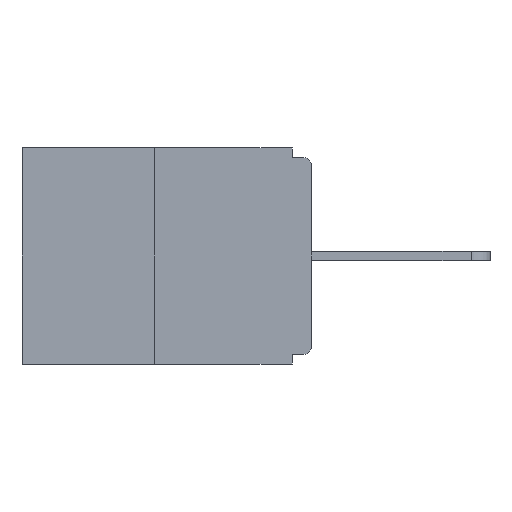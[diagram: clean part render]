
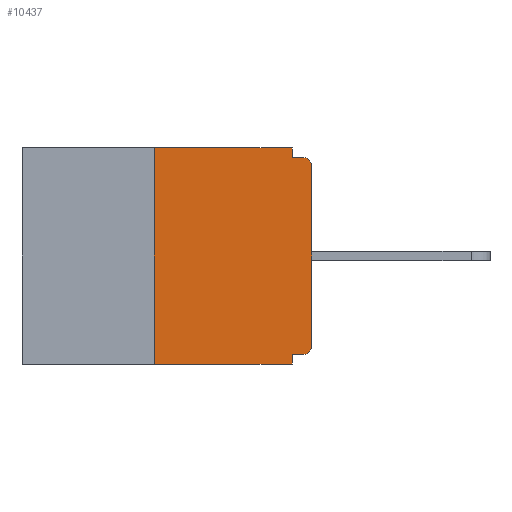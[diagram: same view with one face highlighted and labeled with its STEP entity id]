
A CAD part, left-side view. The second image highlights one B-rep face of the part: STEP entity #10437.
In plain terms, the highlighted planar face has unit normal (-1, 0, 0).
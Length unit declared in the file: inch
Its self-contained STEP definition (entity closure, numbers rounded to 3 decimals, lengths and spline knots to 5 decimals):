
#19 = ORIENTED_EDGE ( 'NONE', *, *, #15145, .T. ) ;
#42 = ORIENTED_EDGE ( 'NONE', *, *, #15051, .T. ) ;
#130 = ORIENTED_EDGE ( 'NONE', *, *, #1402, .F. ) ;
#151 = ORIENTED_EDGE ( 'NONE', *, *, #12578, .F. ) ;
#201 = CARTESIAN_POINT ( 'NONE',  ( 0., 0., -0.03 ) ) ;
#251 = CARTESIAN_POINT ( 'NONE',  ( 0., 0., -0.015 ) ) ;
#617 = VECTOR ( 'NONE', #9192, 39.37008 ) ;
#1059 = ORIENTED_EDGE ( 'NONE', *, *, #19638, .F. ) ;
#1088 = CARTESIAN_POINT ( 'NONE',  ( 0., 0., -0.313 ) ) ;
#1100 = VERTEX_POINT ( 'NONE', #18998 ) ;
#1280 = VERTEX_POINT ( 'NONE', #12153 ) ;
#1402 = EDGE_CURVE ( 'NONE', #17087, #4233, #5703, .T. ) ;
#1859 = DIRECTION ( 'NONE',  ( 0., 0., -1. ) ) ;
#1867 = DIRECTION ( 'NONE',  ( -1., 0., 0. ) ) ;
#1935 = CARTESIAN_POINT ( 'NONE',  ( 0., 0.015, -0.313 ) ) ;
#2205 = CARTESIAN_POINT ( 'NONE',  ( 0., 0.015, -0.03 ) ) ;
#2470 = PLANE ( 'NONE',  #6472 ) ;
#2731 = ORIENTED_EDGE ( 'NONE', *, *, #7790, .T. ) ;
#3092 = CIRCLE ( 'NONE', #11949, 0.015 ) ;
#3506 = CARTESIAN_POINT ( 'NONE',  ( 0., 0.031, 0. ) ) ;
#3685 = VECTOR ( 'NONE', #6808, 39.37008 ) ;
#3762 = EDGE_CURVE ( 'NONE', #1280, #19052, #5853, .T. ) ;
#3929 = DIRECTION ( 'NONE',  ( 0., 0., -1. ) ) ;
#3944 = VECTOR ( 'NONE', #5799, 39.37008 ) ;
#4233 = VERTEX_POINT ( 'NONE', #14925 ) ;
#4263 = DIRECTION ( 'NONE',  ( 0., 0., -1. ) ) ;
#4659 = CARTESIAN_POINT ( 'NONE',  ( 0., 0.25, 0. ) ) ;
#5539 = VERTEX_POINT ( 'NONE', #1088 ) ;
#5685 = LINE ( 'NONE', #17289, #617 ) ;
#5703 = LINE ( 'NONE', #251, #9600 ) ;
#5799 = DIRECTION ( 'NONE',  ( 0., -1., 0. ) ) ;
#5853 = LINE ( 'NONE', #10590, #9749 ) ;
#6281 = VECTOR ( 'NONE', #19668, 39.37008 ) ;
#6472 = AXIS2_PLACEMENT_3D ( 'NONE', #20515, #14186, #4263 ) ;
#6808 = DIRECTION ( 'NONE',  ( 0., 0., -1. ) ) ;
#7246 = CIRCLE ( 'NONE', #17471, 0.015 ) ;
#7374 = EDGE_CURVE ( 'NONE', #8950, #9987, #12668, .T. ) ;
#7462 = CARTESIAN_POINT ( 'NONE',  ( 0., 0.46, 0. ) ) ;
#7615 = LINE ( 'NONE', #3506, #3685 ) ;
#7790 = EDGE_CURVE ( 'NONE', #8950, #20826, #12431, .T. ) ;
#8315 = EDGE_CURVE ( 'NONE', #1280, #5539, #3092, .T. ) ;
#8382 = ORIENTED_EDGE ( 'NONE', *, *, #7374, .F. ) ;
#8950 = VERTEX_POINT ( 'NONE', #19657 ) ;
#9192 = DIRECTION ( 'NONE',  ( 0., 0., 1. ) ) ;
#9600 = VECTOR ( 'NONE', #20470, 39.37008 ) ;
#9749 = VECTOR ( 'NONE', #10820, 39.37008 ) ;
#9987 = VERTEX_POINT ( 'NONE', #4659 ) ;
#10011 = CARTESIAN_POINT ( 'NONE',  ( 0., 0.031, -0.343 ) ) ;
#10437 = ADVANCED_FACE ( 'NONE', ( #19872 ), #2470, .F. ) ;
#10590 = CARTESIAN_POINT ( 'NONE',  ( 0., 0., -0.328 ) ) ;
#10701 = LINE ( 'NONE', #10011, #6281 ) ;
#10724 = ORIENTED_EDGE ( 'NONE', *, *, #21167, .F. ) ;
#10820 = DIRECTION ( 'NONE',  ( 0., 1., 0. ) ) ;
#11164 = VECTOR ( 'NONE', #19238, 39.37008 ) ;
#11949 = AXIS2_PLACEMENT_3D ( 'NONE', #1935, #1867, #1859 ) ;
#11988 = ORIENTED_EDGE ( 'NONE', *, *, #8315, .T. ) ;
#12153 = CARTESIAN_POINT ( 'NONE',  ( 0., 0.015, -0.328 ) ) ;
#12229 = CARTESIAN_POINT ( 'NONE',  ( 0., 0.031, -0.015 ) ) ;
#12431 = LINE ( 'NONE', #18201, #20487 ) ;
#12578 = EDGE_CURVE ( 'NONE', #1100, #17087, #7615, .T. ) ;
#12668 = LINE ( 'NONE', #19597, #11164 ) ;
#13865 = DIRECTION ( 'NONE',  ( -1., 0., 0. ) ) ;
#14186 = DIRECTION ( 'NONE',  ( 1., 0., 0. ) ) ;
#14925 = CARTESIAN_POINT ( 'NONE',  ( 0., 0.015, -0.015 ) ) ;
#15051 = EDGE_CURVE ( 'NONE', #20065, #4233, #7246, .T. ) ;
#15145 = EDGE_CURVE ( 'NONE', #5539, #20065, #5685, .T. ) ;
#15616 = CARTESIAN_POINT ( 'NONE',  ( 0., 0.031, -0.343 ) ) ;
#17070 = LINE ( 'NONE', #7462, #3944 ) ;
#17087 = VERTEX_POINT ( 'NONE', #12229 ) ;
#17289 = CARTESIAN_POINT ( 'NONE',  ( 0., 0., 0. ) ) ;
#17471 = AXIS2_PLACEMENT_3D ( 'NONE', #2205, #13865, #3929 ) ;
#18201 = CARTESIAN_POINT ( 'NONE',  ( 0., 0.46, -0.343 ) ) ;
#18288 = DIRECTION ( 'NONE',  ( 0., -1., 0. ) ) ;
#18998 = CARTESIAN_POINT ( 'NONE',  ( 0., 0.031, 0. ) ) ;
#19052 = VERTEX_POINT ( 'NONE', #19486 ) ;
#19238 = DIRECTION ( 'NONE',  ( 0., 0., 1. ) ) ;
#19486 = CARTESIAN_POINT ( 'NONE',  ( 0., 0.031, -0.328 ) ) ;
#19597 = CARTESIAN_POINT ( 'NONE',  ( 0., 0.25, 0. ) ) ;
#19638 = EDGE_CURVE ( 'NONE', #9987, #1100, #17070, .T. ) ;
#19657 = CARTESIAN_POINT ( 'NONE',  ( 0., 0.25, -0.343 ) ) ;
#19668 = DIRECTION ( 'NONE',  ( 0., 0., -1. ) ) ;
#19872 = FACE_OUTER_BOUND ( 'NONE', #21291, .T. ) ;
#20065 = VERTEX_POINT ( 'NONE', #201 ) ;
#20087 = ORIENTED_EDGE ( 'NONE', *, *, #3762, .F. ) ;
#20470 = DIRECTION ( 'NONE',  ( 0., -1., 0. ) ) ;
#20487 = VECTOR ( 'NONE', #18288, 39.37008 ) ;
#20515 = CARTESIAN_POINT ( 'NONE',  ( 0., 0.46, 0. ) ) ;
#20826 = VERTEX_POINT ( 'NONE', #15616 ) ;
#21167 = EDGE_CURVE ( 'NONE', #19052, #20826, #10701, .T. ) ;
#21291 = EDGE_LOOP ( 'NONE', ( #1059, #8382, #2731, #10724, #20087, #11988, #19, #42, #130, #151 ) ) ;
